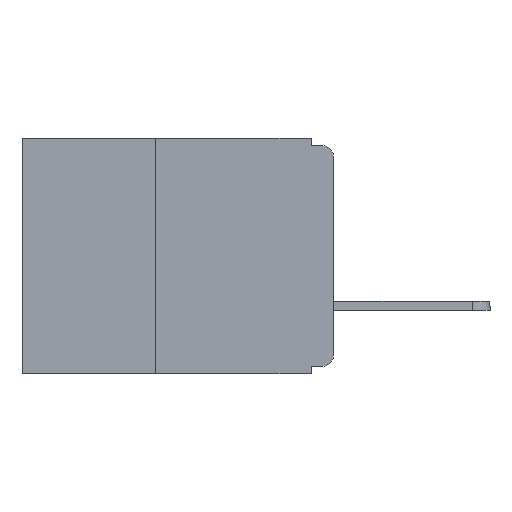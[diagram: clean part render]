
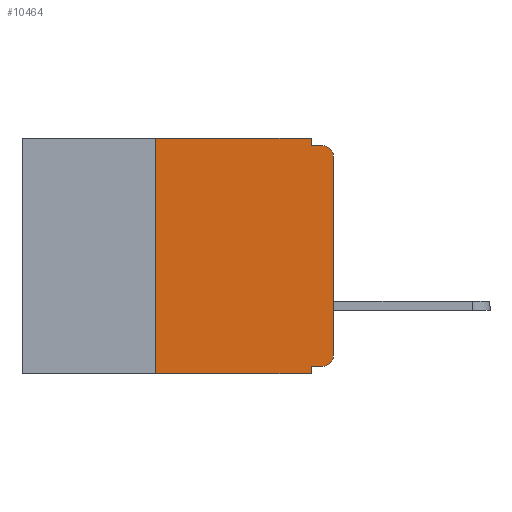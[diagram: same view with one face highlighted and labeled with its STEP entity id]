
A CAD part, left-side view. The second image highlights one B-rep face of the part: STEP entity #10464.
In plain terms, the highlighted planar face has unit normal (-1, 0, 0).
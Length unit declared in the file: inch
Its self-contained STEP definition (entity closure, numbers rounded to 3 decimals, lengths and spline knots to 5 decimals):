
#225 = CARTESIAN_POINT ( 'NONE',  ( 0., 0.031, -0.01 ) ) ;
#563 = DIRECTION ( 'NONE',  ( 0., 0., -1. ) ) ;
#631 = ORIENTED_EDGE ( 'NONE', *, *, #12952, .F. ) ;
#679 = EDGE_CURVE ( 'NONE', #9713, #13023, #13407, .T. ) ;
#710 = ORIENTED_EDGE ( 'NONE', *, *, #2308, .T. ) ;
#920 = CARTESIAN_POINT ( 'NONE',  ( 0., 0.031, -0.33 ) ) ;
#1052 = ORIENTED_EDGE ( 'NONE', *, *, #10055, .F. ) ;
#1367 = VECTOR ( 'NONE', #1737, 39.37008 ) ;
#1501 = ORIENTED_EDGE ( 'NONE', *, *, #4395, .T. ) ;
#1553 = CARTESIAN_POINT ( 'NONE',  ( 0., 0., -0.025 ) ) ;
#1637 = LINE ( 'NONE', #1823, #1367 ) ;
#1737 = DIRECTION ( 'NONE',  ( 0., -1., 0. ) ) ;
#1823 = CARTESIAN_POINT ( 'NONE',  ( 0., 0., -0.01 ) ) ;
#2018 = CARTESIAN_POINT ( 'NONE',  ( 0., 0.031, 0. ) ) ;
#2046 = AXIS2_PLACEMENT_3D ( 'NONE', #13794, #13635, #13588 ) ;
#2308 = EDGE_CURVE ( 'NONE', #17312, #10299, #4013, .T. ) ;
#2919 = EDGE_LOOP ( 'NONE', ( #12578, #1501, #3539, #4974, #7491, #631, #16842, #1052, #6304, #710 ) ) ;
#3397 = DIRECTION ( 'NONE',  ( 0., 0., 1. ) ) ;
#3453 = VERTEX_POINT ( 'NONE', #1553 ) ;
#3539 = ORIENTED_EDGE ( 'NONE', *, *, #15928, .F. ) ;
#3682 = CARTESIAN_POINT ( 'NONE',  ( 0., 0.25, -0.33 ) ) ;
#4013 = CIRCLE ( 'NONE', #6078, 0.015 ) ;
#4143 = CARTESIAN_POINT ( 'NONE',  ( 0., 0.25, 0. ) ) ;
#4395 = EDGE_CURVE ( 'NONE', #3453, #7444, #17580, .T. ) ;
#4974 = ORIENTED_EDGE ( 'NONE', *, *, #9381, .F. ) ;
#5313 = AXIS2_PLACEMENT_3D ( 'NONE', #9726, #9722, #9697 ) ;
#5472 = VERTEX_POINT ( 'NONE', #7256 ) ;
#5786 = VERTEX_POINT ( 'NONE', #14708 ) ;
#6078 = AXIS2_PLACEMENT_3D ( 'NONE', #8487, #8187, #15909 ) ;
#6304 = ORIENTED_EDGE ( 'NONE', *, *, #14109, .F. ) ;
#6324 = VERTEX_POINT ( 'NONE', #13422 ) ;
#6825 = VECTOR ( 'NONE', #9451, 39.37008 ) ;
#6985 = LINE ( 'NONE', #9169, #6825 ) ;
#7256 = CARTESIAN_POINT ( 'NONE',  ( 0., 0.031, -0.32 ) ) ;
#7444 = VERTEX_POINT ( 'NONE', #13161 ) ;
#7491 = ORIENTED_EDGE ( 'NONE', *, *, #679, .F. ) ;
#8187 = DIRECTION ( 'NONE',  ( -1., 0., 0. ) ) ;
#8344 = VECTOR ( 'NONE', #17022, 39.37008 ) ;
#8458 = LINE ( 'NONE', #17124, #8344 ) ;
#8487 = CARTESIAN_POINT ( 'NONE',  ( 0., 0.015, -0.305 ) ) ;
#9169 = CARTESIAN_POINT ( 'NONE',  ( 0., 0.437, -0.33 ) ) ;
#9381 = EDGE_CURVE ( 'NONE', #13023, #10065, #17163, .T. ) ;
#9395 = VECTOR ( 'NONE', #15979, 39.37008 ) ;
#9451 = DIRECTION ( 'NONE',  ( 0., -1., 0. ) ) ;
#9697 = DIRECTION ( 'NONE',  ( 0., 0., -1. ) ) ;
#9713 = VERTEX_POINT ( 'NONE', #4143 ) ;
#9722 = DIRECTION ( 'NONE',  ( 1., 0., 0. ) ) ;
#9726 = CARTESIAN_POINT ( 'NONE',  ( 0., 0.437, 0. ) ) ;
#9758 = LINE ( 'NONE', #15670, #9395 ) ;
#10055 = EDGE_CURVE ( 'NONE', #5472, #6324, #13402, .T. ) ;
#10065 = VERTEX_POINT ( 'NONE', #225 ) ;
#10299 = VERTEX_POINT ( 'NONE', #14064 ) ;
#10422 = PLANE ( 'NONE',  #5313 ) ;
#10464 = ADVANCED_FACE ( 'NONE', ( #10600 ), #10422, .F. ) ;
#10600 = FACE_OUTER_BOUND ( 'NONE', #2919, .T. ) ;
#12578 = ORIENTED_EDGE ( 'NONE', *, *, #17365, .T. ) ;
#12686 = CARTESIAN_POINT ( 'NONE',  ( 0., 0.437, 0. ) ) ;
#12952 = EDGE_CURVE ( 'NONE', #5786, #9713, #15483, .T. ) ;
#13023 = VERTEX_POINT ( 'NONE', #2018 ) ;
#13047 = VECTOR ( 'NONE', #563, 39.37008 ) ;
#13127 = VECTOR ( 'NONE', #17977, 39.37008 ) ;
#13161 = CARTESIAN_POINT ( 'NONE',  ( 0., 0.015, -0.01 ) ) ;
#13402 = LINE ( 'NONE', #920, #13047 ) ;
#13407 = LINE ( 'NONE', #12686, #13127 ) ;
#13422 = CARTESIAN_POINT ( 'NONE',  ( 0., 0.031, -0.33 ) ) ;
#13588 = DIRECTION ( 'NONE',  ( 0., 0., -1. ) ) ;
#13635 = DIRECTION ( 'NONE',  ( -1., 0., 0. ) ) ;
#13794 = CARTESIAN_POINT ( 'NONE',  ( 0., 0.015, -0.025 ) ) ;
#14064 = CARTESIAN_POINT ( 'NONE',  ( 0., 0., -0.305 ) ) ;
#14109 = EDGE_CURVE ( 'NONE', #17312, #5472, #9758, .T. ) ;
#14708 = CARTESIAN_POINT ( 'NONE',  ( 0., 0.25, -0.33 ) ) ;
#15200 = DIRECTION ( 'NONE',  ( 0., 0., -1. ) ) ;
#15404 = CARTESIAN_POINT ( 'NONE',  ( 0., 0.031, 0. ) ) ;
#15448 = VECTOR ( 'NONE', #3397, 39.37008 ) ;
#15483 = LINE ( 'NONE', #3682, #15448 ) ;
#15670 = CARTESIAN_POINT ( 'NONE',  ( 0., 0., -0.32 ) ) ;
#15909 = DIRECTION ( 'NONE',  ( 0., 0., -1. ) ) ;
#15928 = EDGE_CURVE ( 'NONE', #10065, #7444, #1637, .T. ) ;
#15979 = DIRECTION ( 'NONE',  ( 0., 1., 0. ) ) ;
#16842 = ORIENTED_EDGE ( 'NONE', *, *, #17622, .T. ) ;
#17022 = DIRECTION ( 'NONE',  ( 0., 0., 1. ) ) ;
#17115 = VECTOR ( 'NONE', #15200, 39.37008 ) ;
#17124 = CARTESIAN_POINT ( 'NONE',  ( 0., 0., 0. ) ) ;
#17163 = LINE ( 'NONE', #15404, #17115 ) ;
#17312 = VERTEX_POINT ( 'NONE', #18558 ) ;
#17365 = EDGE_CURVE ( 'NONE', #10299, #3453, #8458, .T. ) ;
#17580 = CIRCLE ( 'NONE', #2046, 0.015 ) ;
#17622 = EDGE_CURVE ( 'NONE', #5786, #6324, #6985, .T. ) ;
#17977 = DIRECTION ( 'NONE',  ( 0., -1., 0. ) ) ;
#18558 = CARTESIAN_POINT ( 'NONE',  ( 0., 0.015, -0.32 ) ) ;
